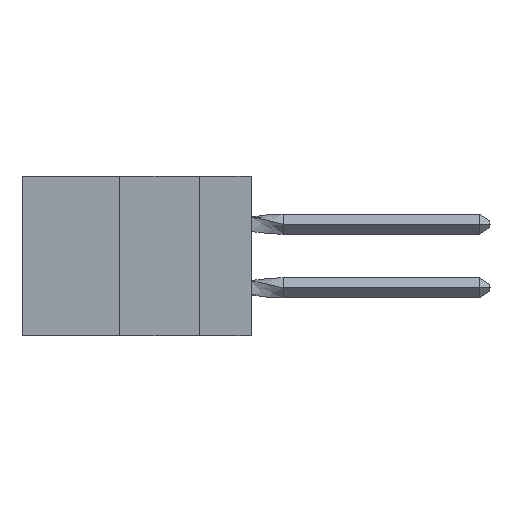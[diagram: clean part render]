
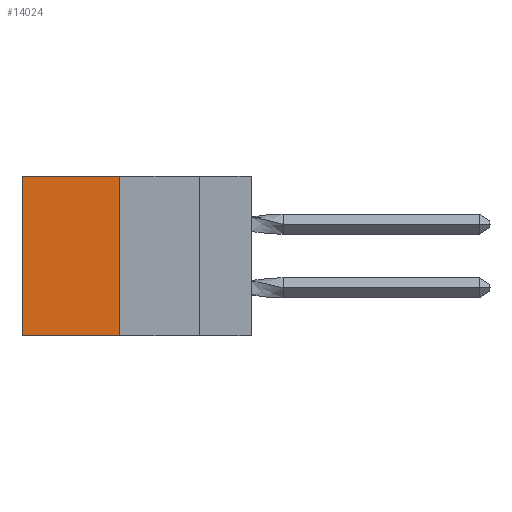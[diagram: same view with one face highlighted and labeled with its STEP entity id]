
A CAD part, left-side view. The second image highlights one B-rep face of the part: STEP entity #14024.
In plain terms, the highlighted planar face has unit normal (-1, 0, 0).
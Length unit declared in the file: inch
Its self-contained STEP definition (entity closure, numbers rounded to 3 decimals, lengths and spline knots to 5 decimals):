
#540 = CARTESIAN_POINT ( 'NONE',  ( 0.305, 0.72, -0.5 ) ) ;
#4368 = ORIENTED_EDGE ( 'NONE', *, *, #8994, .T. ) ;
#4635 = VECTOR ( 'NONE', #9311, 39.37008 ) ;
#4766 = CARTESIAN_POINT ( 'NONE',  ( 0.305, 0.413, 0. ) ) ;
#5527 = CARTESIAN_POINT ( 'NONE',  ( 0.305, 0.413, 0. ) ) ;
#5687 = VERTEX_POINT ( 'NONE', #6785 ) ;
#5851 = CARTESIAN_POINT ( 'NONE',  ( 0.305, 0.413, -0.5 ) ) ;
#6479 = VECTOR ( 'NONE', #9426, 39.37008 ) ;
#6578 = DIRECTION ( 'NONE',  ( 0., 1., 0. ) ) ;
#6785 = CARTESIAN_POINT ( 'NONE',  ( 0.305, 0.72, -0.5 ) ) ;
#7133 = FACE_OUTER_BOUND ( 'NONE', #14038, .T. ) ;
#7705 = CARTESIAN_POINT ( 'NONE',  ( 0.305, 0.413, -0.5 ) ) ;
#8100 = PLANE ( 'NONE',  #16564 ) ;
#8345 = VERTEX_POINT ( 'NONE', #5527 ) ;
#8994 = EDGE_CURVE ( 'NONE', #15574, #5687, #18527, .T. ) ;
#9311 = DIRECTION ( 'NONE',  ( 0., 1., 0. ) ) ;
#9426 = DIRECTION ( 'NONE',  ( 0., 0., -1. ) ) ;
#11769 = DIRECTION ( 'NONE',  ( 1., 0., 0. ) ) ;
#13330 = ORIENTED_EDGE ( 'NONE', *, *, #22198, .F. ) ;
#13463 = LINE ( 'NONE', #7705, #15400 ) ;
#13473 = EDGE_CURVE ( 'NONE', #14751, #5687, #21101, .T. ) ;
#13525 = ORIENTED_EDGE ( 'NONE', *, *, #17307, .T. ) ;
#14024 = ADVANCED_FACE ( 'NONE', ( #7133 ), #8100, .F. ) ;
#14038 = EDGE_LOOP ( 'NONE', ( #4368, #16401, #13330, #13525 ) ) ;
#14207 = VECTOR ( 'NONE', #6578, 39.37008 ) ;
#14665 = DIRECTION ( 'NONE',  ( 0., 0., -1. ) ) ;
#14751 = VERTEX_POINT ( 'NONE', #15456 ) ;
#15400 = VECTOR ( 'NONE', #14665, 39.37008 ) ;
#15456 = CARTESIAN_POINT ( 'NONE',  ( 0.305, 0.413, -0.5 ) ) ;
#15574 = VERTEX_POINT ( 'NONE', #18603 ) ;
#16401 = ORIENTED_EDGE ( 'NONE', *, *, #13473, .F. ) ;
#16564 = AXIS2_PLACEMENT_3D ( 'NONE', #18788, #11769, #20483 ) ;
#17307 = EDGE_CURVE ( 'NONE', #8345, #15574, #18955, .T. ) ;
#18527 = LINE ( 'NONE', #540, #6479 ) ;
#18603 = CARTESIAN_POINT ( 'NONE',  ( 0.305, 0.72, 0. ) ) ;
#18788 = CARTESIAN_POINT ( 'NONE',  ( 0.305, 0.413, -0.5 ) ) ;
#18955 = LINE ( 'NONE', #4766, #14207 ) ;
#20483 = DIRECTION ( 'NONE',  ( 0., 0., -1. ) ) ;
#21101 = LINE ( 'NONE', #5851, #4635 ) ;
#22198 = EDGE_CURVE ( 'NONE', #8345, #14751, #13463, .T. ) ;
